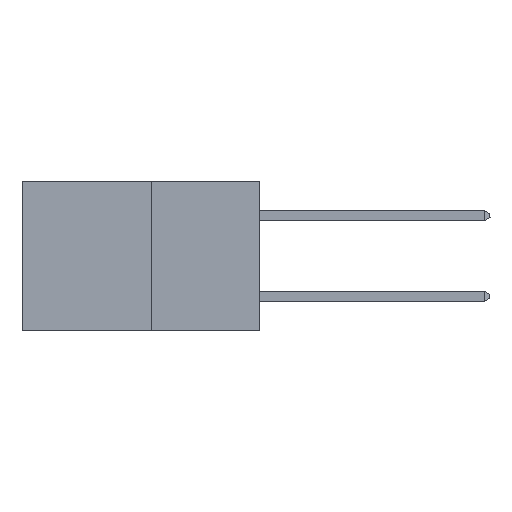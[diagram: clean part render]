
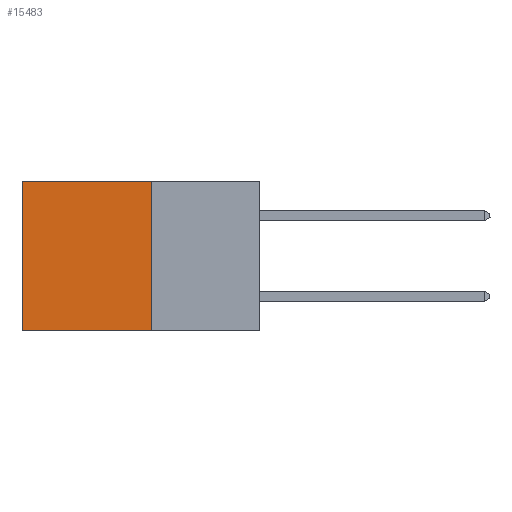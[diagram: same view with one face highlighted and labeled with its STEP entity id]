
A CAD part, left-side view. The second image highlights one B-rep face of the part: STEP entity #15483.
In plain terms, the highlighted planar face has unit normal (-1, 0, 0).
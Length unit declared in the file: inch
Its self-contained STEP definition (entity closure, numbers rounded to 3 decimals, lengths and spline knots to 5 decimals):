
#1094 = VECTOR ( 'NONE', #20239, 39.37008 ) ;
#1714 = DIRECTION ( 'NONE',  ( 0., 0., -1. ) ) ;
#2541 = VECTOR ( 'NONE', #25401, 39.37008 ) ;
#2907 = ORIENTED_EDGE ( 'NONE', *, *, #20228, .F. ) ;
#3213 = LINE ( 'NONE', #8057, #2541 ) ;
#4036 = EDGE_CURVE ( 'NONE', #27518, #6883, #7507, .T. ) ;
#6819 = AXIS2_PLACEMENT_3D ( 'NONE', #27674, #14738, #1714 ) ;
#6883 = VERTEX_POINT ( 'NONE', #9857 ) ;
#6928 = LINE ( 'NONE', #13078, #22981 ) ;
#7507 = LINE ( 'NONE', #20665, #1094 ) ;
#7723 = CARTESIAN_POINT ( 'NONE',  ( 0.277, 0.59, 0. ) ) ;
#8057 = CARTESIAN_POINT ( 'NONE',  ( 0.277, 0.27, -0.37 ) ) ;
#8709 = CARTESIAN_POINT ( 'NONE',  ( 0.277, 0.27, -0.37 ) ) ;
#8902 = EDGE_CURVE ( 'NONE', #23462, #10460, #13236, .T. ) ;
#9857 = CARTESIAN_POINT ( 'NONE',  ( 0.277, 0.59, -0.37 ) ) ;
#10460 = VERTEX_POINT ( 'NONE', #8709 ) ;
#11141 = ORIENTED_EDGE ( 'NONE', *, *, #19858, .T. ) ;
#11748 = ORIENTED_EDGE ( 'NONE', *, *, #8902, .F. ) ;
#12548 = PLANE ( 'NONE',  #6819 ) ;
#13078 = CARTESIAN_POINT ( 'NONE',  ( 0.277, 0.27, 0. ) ) ;
#13236 = LINE ( 'NONE', #22781, #24125 ) ;
#14738 = DIRECTION ( 'NONE',  ( 1., 0., 0. ) ) ;
#15201 = ORIENTED_EDGE ( 'NONE', *, *, #4036, .T. ) ;
#15483 = ADVANCED_FACE ( 'NONE', ( #17151 ), #12548, .F. ) ;
#16649 = EDGE_LOOP ( 'NONE', ( #15201, #2907, #11748, #11141 ) ) ;
#17151 = FACE_OUTER_BOUND ( 'NONE', #16649, .T. ) ;
#19858 = EDGE_CURVE ( 'NONE', #23462, #27518, #6928, .T. ) ;
#20228 = EDGE_CURVE ( 'NONE', #10460, #6883, #3213, .T. ) ;
#20239 = DIRECTION ( 'NONE',  ( 0., 0., -1. ) ) ;
#20665 = CARTESIAN_POINT ( 'NONE',  ( 0.277, 0.59, -0.37 ) ) ;
#21402 = CARTESIAN_POINT ( 'NONE',  ( 0.277, 0.27, 0. ) ) ;
#22511 = DIRECTION ( 'NONE',  ( 0., 0., -1. ) ) ;
#22781 = CARTESIAN_POINT ( 'NONE',  ( 0.277, 0.27, -0.37 ) ) ;
#22981 = VECTOR ( 'NONE', #24020, 39.37008 ) ;
#23462 = VERTEX_POINT ( 'NONE', #21402 ) ;
#24020 = DIRECTION ( 'NONE',  ( 0., 1., 0. ) ) ;
#24125 = VECTOR ( 'NONE', #22511, 39.37008 ) ;
#25401 = DIRECTION ( 'NONE',  ( 0., 1., 0. ) ) ;
#27518 = VERTEX_POINT ( 'NONE', #7723 ) ;
#27674 = CARTESIAN_POINT ( 'NONE',  ( 0.277, 0.27, -0.37 ) ) ;
